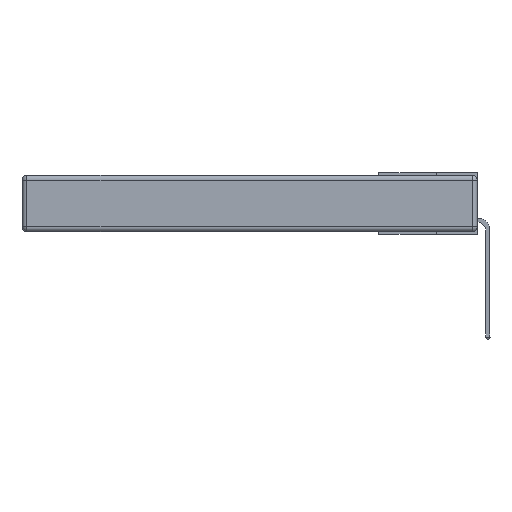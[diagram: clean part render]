
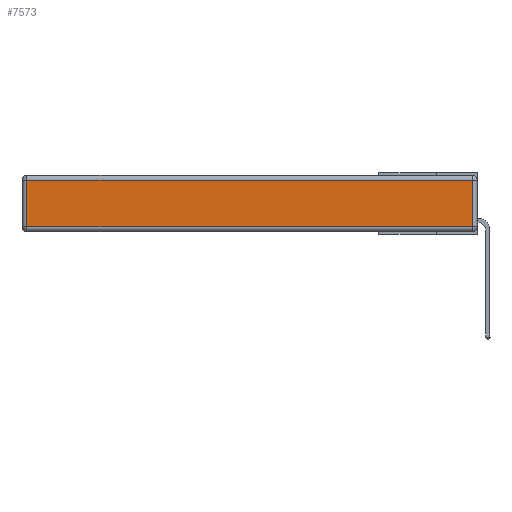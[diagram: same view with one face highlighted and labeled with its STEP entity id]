
A CAD part, left-side view. The second image highlights one B-rep face of the part: STEP entity #7573.
In plain terms, the highlighted planar face has unit normal (-1, 0, 0).
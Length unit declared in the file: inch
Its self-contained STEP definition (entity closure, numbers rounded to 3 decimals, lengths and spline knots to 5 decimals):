
#835 = EDGE_CURVE ( 'NONE', #14726, #5141, #1687, .T. ) ;
#856 = CARTESIAN_POINT ( 'NONE',  ( 0., 0., -0.343 ) ) ;
#1245 = VECTOR ( 'NONE', #4083, 39.37008 ) ;
#1423 = CARTESIAN_POINT ( 'NONE',  ( 0., 2.72, -0.03 ) ) ;
#1467 = CARTESIAN_POINT ( 'NONE',  ( 0., 0.03, -0.343 ) ) ;
#1687 = LINE ( 'NONE', #1467, #18730 ) ;
#2650 = ORIENTED_EDGE ( 'NONE', *, *, #12940, .T. ) ;
#2966 = DIRECTION ( 'NONE',  ( 0., 0., 1. ) ) ;
#3272 = ORIENTED_EDGE ( 'NONE', *, *, #11176, .T. ) ;
#3649 = DIRECTION ( 'NONE',  ( 0., 0., 1. ) ) ;
#4083 = DIRECTION ( 'NONE',  ( 0., -1., 0. ) ) ;
#5141 = VERTEX_POINT ( 'NONE', #15202 ) ;
#5329 = CARTESIAN_POINT ( 'NONE',  ( 0., 2.75, -0.03 ) ) ;
#7160 = CARTESIAN_POINT ( 'NONE',  ( 0., 0.03, -0.313 ) ) ;
#7573 = ADVANCED_FACE ( 'NONE', ( #11358 ), #15652, .T. ) ;
#7596 = VECTOR ( 'NONE', #17876, 39.37008 ) ;
#8427 = VERTEX_POINT ( 'NONE', #1423 ) ;
#9404 = AXIS2_PLACEMENT_3D ( 'NONE', #856, #11154, #3649 ) ;
#9790 = ORIENTED_EDGE ( 'NONE', *, *, #10459, .T. ) ;
#10007 = CARTESIAN_POINT ( 'NONE',  ( 0., 2.72, -0.313 ) ) ;
#10459 = EDGE_CURVE ( 'NONE', #5141, #8427, #12774, .T. ) ;
#10892 = EDGE_LOOP ( 'NONE', ( #2650, #16464, #9790, #3272 ) ) ;
#11154 = DIRECTION ( 'NONE',  ( -1., 0., 0. ) ) ;
#11176 = EDGE_CURVE ( 'NONE', #8427, #15141, #16496, .T. ) ;
#11358 = FACE_OUTER_BOUND ( 'NONE', #10892, .T. ) ;
#12062 = VECTOR ( 'NONE', #12766, 39.37008 ) ;
#12766 = DIRECTION ( 'NONE',  ( 0., 1., 0. ) ) ;
#12774 = LINE ( 'NONE', #5329, #12062 ) ;
#12940 = EDGE_CURVE ( 'NONE', #15141, #14726, #18540, .T. ) ;
#14726 = VERTEX_POINT ( 'NONE', #7160 ) ;
#15141 = VERTEX_POINT ( 'NONE', #10007 ) ;
#15202 = CARTESIAN_POINT ( 'NONE',  ( 0., 0.03, -0.03 ) ) ;
#15652 = PLANE ( 'NONE',  #9404 ) ;
#16464 = ORIENTED_EDGE ( 'NONE', *, *, #835, .T. ) ;
#16496 = LINE ( 'NONE', #18981, #7596 ) ;
#17876 = DIRECTION ( 'NONE',  ( 0., 0., -1. ) ) ;
#18540 = LINE ( 'NONE', #19082, #1245 ) ;
#18730 = VECTOR ( 'NONE', #2966, 39.37008 ) ;
#18981 = CARTESIAN_POINT ( 'NONE',  ( 0., 2.72, -0.343 ) ) ;
#19082 = CARTESIAN_POINT ( 'NONE',  ( 0., 0., -0.313 ) ) ;
